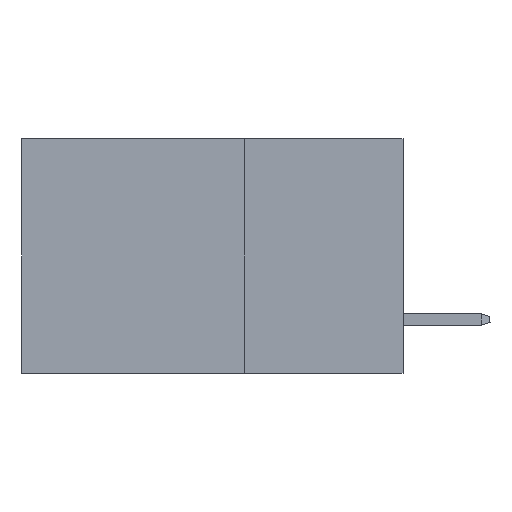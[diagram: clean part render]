
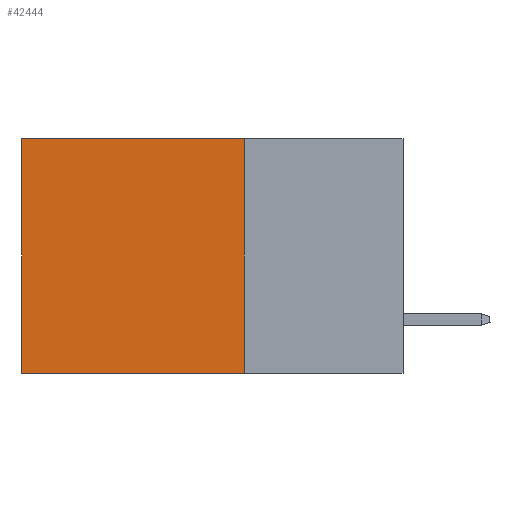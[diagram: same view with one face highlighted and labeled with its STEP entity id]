
A CAD part, left-side view. The second image highlights one B-rep face of the part: STEP entity #42444.
In plain terms, the highlighted planar face has unit normal (-1, 0, 0).
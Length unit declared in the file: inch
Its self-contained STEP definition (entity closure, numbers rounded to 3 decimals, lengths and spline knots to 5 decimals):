
#411 = CARTESIAN_POINT ( 'NONE',  ( 0.2875, 0.25, 0. ) ) ;
#1223 = VECTOR ( 'NONE', #45197, 39.37008 ) ;
#5598 = CARTESIAN_POINT ( 'NONE',  ( 0.2875, 0.6, 0. ) ) ;
#6092 = ORIENTED_EDGE ( 'NONE', *, *, #9610, .F. ) ;
#6169 = CARTESIAN_POINT ( 'NONE',  ( 0.2875, 0.6, 0. ) ) ;
#7695 = CARTESIAN_POINT ( 'NONE',  ( 0.2875, 0.25, 0. ) ) ;
#8204 = CARTESIAN_POINT ( 'NONE',  ( 0.2875, 0.6, -0.37 ) ) ;
#9456 = LINE ( 'NONE', #5598, #12143 ) ;
#9610 = EDGE_CURVE ( 'NONE', #38816, #45490, #11889, .T. ) ;
#11279 = PLANE ( 'NONE',  #38207 ) ;
#11889 = LINE ( 'NONE', #26627, #13655 ) ;
#12143 = VECTOR ( 'NONE', #34573, 39.37008 ) ;
#13655 = VECTOR ( 'NONE', #22514, 39.37008 ) ;
#16785 = CARTESIAN_POINT ( 'NONE',  ( 0.2875, 0.25, 0. ) ) ;
#19523 = EDGE_LOOP ( 'NONE', ( #41643, #30166, #6092, #41109 ) ) ;
#19600 = CARTESIAN_POINT ( 'NONE',  ( 0.2875, 0.25, -0.37 ) ) ;
#22514 = DIRECTION ( 'NONE',  ( 0., 0., -1. ) ) ;
#23497 = EDGE_CURVE ( 'NONE', #45490, #27220, #34106, .T. ) ;
#24506 = DIRECTION ( 'NONE',  ( 0., 1., 0. ) ) ;
#26287 = EDGE_CURVE ( 'NONE', #38816, #47078, #35151, .T. ) ;
#26627 = CARTESIAN_POINT ( 'NONE',  ( 0.2875, 0.25, 0. ) ) ;
#27220 = VERTEX_POINT ( 'NONE', #8204 ) ;
#28402 = VECTOR ( 'NONE', #24506, 39.37008 ) ;
#30166 = ORIENTED_EDGE ( 'NONE', *, *, #23497, .F. ) ;
#34106 = LINE ( 'NONE', #19600, #1223 ) ;
#34573 = DIRECTION ( 'NONE',  ( 0., 0., -1. ) ) ;
#35151 = LINE ( 'NONE', #16785, #28402 ) ;
#35569 = CARTESIAN_POINT ( 'NONE',  ( 0.2875, 0.25, -0.37 ) ) ;
#37593 = DIRECTION ( 'NONE',  ( 0., 0., -1. ) ) ;
#38207 = AXIS2_PLACEMENT_3D ( 'NONE', #411, #41215, #37593 ) ;
#38635 = EDGE_CURVE ( 'NONE', #47078, #27220, #9456, .T. ) ;
#38816 = VERTEX_POINT ( 'NONE', #7695 ) ;
#41109 = ORIENTED_EDGE ( 'NONE', *, *, #26287, .T. ) ;
#41215 = DIRECTION ( 'NONE',  ( 1., 0., 0. ) ) ;
#41643 = ORIENTED_EDGE ( 'NONE', *, *, #38635, .T. ) ;
#42444 = ADVANCED_FACE ( 'NONE', ( #44357 ), #11279, .F. ) ;
#44357 = FACE_OUTER_BOUND ( 'NONE', #19523, .T. ) ;
#45197 = DIRECTION ( 'NONE',  ( 0., 1., 0. ) ) ;
#45490 = VERTEX_POINT ( 'NONE', #35569 ) ;
#47078 = VERTEX_POINT ( 'NONE', #6169 ) ;
